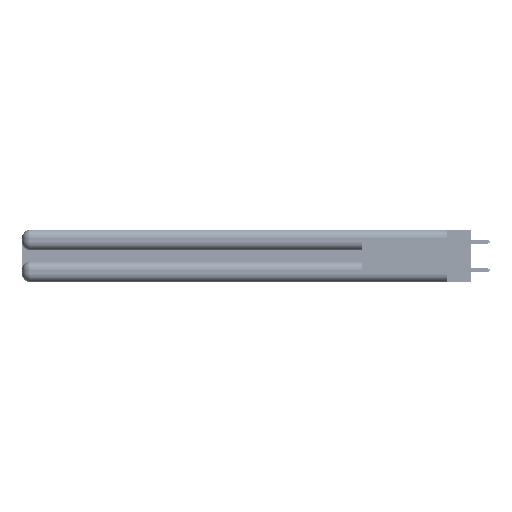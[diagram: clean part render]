
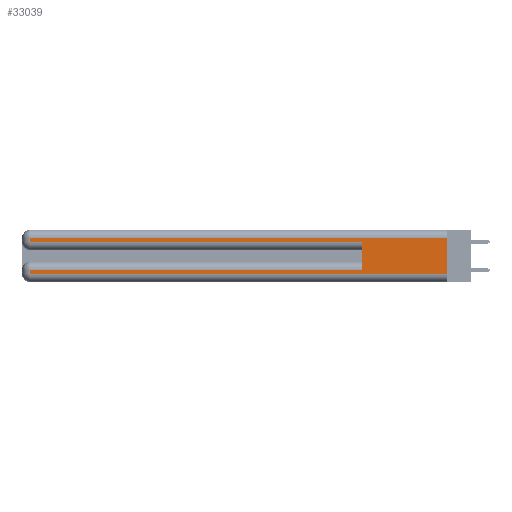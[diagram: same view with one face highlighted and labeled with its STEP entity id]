
A CAD part, left-side view. The second image highlights one B-rep face of the part: STEP entity #33039.
In plain terms, the highlighted planar face has unit normal (-1, 0, 0).
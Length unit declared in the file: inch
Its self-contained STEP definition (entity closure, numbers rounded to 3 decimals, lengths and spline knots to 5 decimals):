
#644 = DIRECTION ( 'NONE',  ( 0., 0., -1. ) ) ;
#691 = VERTEX_POINT ( 'NONE', #37875 ) ;
#998 = VECTOR ( 'NONE', #644, 39.37008 ) ;
#1704 = DIRECTION ( 'NONE',  ( 0., 0., -1. ) ) ;
#1973 = CARTESIAN_POINT ( 'NONE',  ( 0., 0.6, 0.085 ) ) ;
#2137 = CARTESIAN_POINT ( 'NONE',  ( 0., 0., 0.37 ) ) ;
#2329 = PLANE ( 'NONE',  #18157 ) ;
#2964 = CARTESIAN_POINT ( 'NONE',  ( 0., 0., 0.06 ) ) ;
#3198 = VECTOR ( 'NONE', #43396, 39.37008 ) ;
#4211 = VERTEX_POINT ( 'NONE', #26838 ) ;
#4927 = VERTEX_POINT ( 'NONE', #14354 ) ;
#5554 = ORIENTED_EDGE ( 'NONE', *, *, #29229, .T. ) ;
#6200 = EDGE_CURVE ( 'NONE', #4927, #35574, #25321, .T. ) ;
#6906 = VECTOR ( 'NONE', #41886, 39.37008 ) ;
#7474 = VECTOR ( 'NONE', #21379, 39.37008 ) ;
#7859 = EDGE_CURVE ( 'NONE', #49910, #27786, #8196, .T. ) ;
#8196 = LINE ( 'NONE', #25101, #6906 ) ;
#8659 = CARTESIAN_POINT ( 'NONE',  ( 0., 2.94, 0.37 ) ) ;
#9430 = LINE ( 'NONE', #12870, #7474 ) ;
#9996 = DIRECTION ( 'NONE',  ( 1., 0., 0. ) ) ;
#10416 = ORIENTED_EDGE ( 'NONE', *, *, #10869, .F. ) ;
#10869 = EDGE_CURVE ( 'NONE', #4927, #36051, #43702, .T. ) ;
#11335 = ORIENTED_EDGE ( 'NONE', *, *, #46499, .F. ) ;
#12403 = VECTOR ( 'NONE', #1704, 39.37008 ) ;
#12870 = CARTESIAN_POINT ( 'NONE',  ( 0., 0., 0.06 ) ) ;
#13451 = DIRECTION ( 'NONE',  ( 0., 0., 1. ) ) ;
#14354 = CARTESIAN_POINT ( 'NONE',  ( 0., 0., 0.31 ) ) ;
#14579 = CARTESIAN_POINT ( 'NONE',  ( 0., 2.94, 0.31 ) ) ;
#14928 = ORIENTED_EDGE ( 'NONE', *, *, #7859, .T. ) ;
#17277 = LINE ( 'NONE', #8659, #998 ) ;
#18157 = AXIS2_PLACEMENT_3D ( 'NONE', #2137, #9996, #31278 ) ;
#18377 = CARTESIAN_POINT ( 'NONE',  ( 0., 2.94, 0.06 ) ) ;
#20390 = DIRECTION ( 'NONE',  ( 0., 0., -1. ) ) ;
#21379 = DIRECTION ( 'NONE',  ( 0., -1., 0. ) ) ;
#22985 = LINE ( 'NONE', #33536, #52337 ) ;
#23039 = DIRECTION ( 'NONE',  ( 0., -1., 0. ) ) ;
#23845 = ORIENTED_EDGE ( 'NONE', *, *, #33528, .T. ) ;
#24895 = EDGE_CURVE ( 'NONE', #35574, #4211, #22985, .T. ) ;
#25101 = CARTESIAN_POINT ( 'NONE',  ( 0., 0., 0.085 ) ) ;
#25321 = LINE ( 'NONE', #52290, #3198 ) ;
#25607 = ORIENTED_EDGE ( 'NONE', *, *, #38754, .T. ) ;
#26445 = CARTESIAN_POINT ( 'NONE',  ( 0., 0., 0.37 ) ) ;
#26838 = CARTESIAN_POINT ( 'NONE',  ( 0., 2.94, 0.285 ) ) ;
#27786 = VERTEX_POINT ( 'NONE', #51042 ) ;
#29229 = EDGE_CURVE ( 'NONE', #4211, #691, #53080, .T. ) ;
#31278 = DIRECTION ( 'NONE',  ( 0., 0., -1. ) ) ;
#33039 = ADVANCED_FACE ( 'NONE', ( #49948 ), #2329, .F. ) ;
#33528 = EDGE_CURVE ( 'NONE', #27786, #52025, #17277, .T. ) ;
#33536 = CARTESIAN_POINT ( 'NONE',  ( 0., 2.94, 0.37 ) ) ;
#35574 = VERTEX_POINT ( 'NONE', #14579 ) ;
#35591 = ORIENTED_EDGE ( 'NONE', *, *, #6200, .T. ) ;
#35660 = CARTESIAN_POINT ( 'NONE',  ( 0., 0., 0.285 ) ) ;
#35813 = LINE ( 'NONE', #38416, #38411 ) ;
#36051 = VERTEX_POINT ( 'NONE', #2964 ) ;
#36439 = ORIENTED_EDGE ( 'NONE', *, *, #24895, .T. ) ;
#37875 = CARTESIAN_POINT ( 'NONE',  ( 0., 0.6, 0.285 ) ) ;
#38411 = VECTOR ( 'NONE', #13451, 39.37008 ) ;
#38416 = CARTESIAN_POINT ( 'NONE',  ( 0., 0.6, 0.145 ) ) ;
#38754 = EDGE_CURVE ( 'NONE', #52025, #36051, #9430, .T. ) ;
#40065 = VECTOR ( 'NONE', #23039, 39.37008 ) ;
#41886 = DIRECTION ( 'NONE',  ( 0., 1., 0. ) ) ;
#42784 = EDGE_LOOP ( 'NONE', ( #10416, #35591, #36439, #5554, #11335, #14928, #23845, #25607 ) ) ;
#43396 = DIRECTION ( 'NONE',  ( 0., 1., 0. ) ) ;
#43702 = LINE ( 'NONE', #26445, #12403 ) ;
#46499 = EDGE_CURVE ( 'NONE', #49910, #691, #35813, .T. ) ;
#49910 = VERTEX_POINT ( 'NONE', #1973 ) ;
#49948 = FACE_OUTER_BOUND ( 'NONE', #42784, .T. ) ;
#51042 = CARTESIAN_POINT ( 'NONE',  ( 0., 2.94, 0.085 ) ) ;
#52025 = VERTEX_POINT ( 'NONE', #18377 ) ;
#52290 = CARTESIAN_POINT ( 'NONE',  ( 0., 0., 0.31 ) ) ;
#52337 = VECTOR ( 'NONE', #20390, 39.37008 ) ;
#53080 = LINE ( 'NONE', #35660, #40065 ) ;
